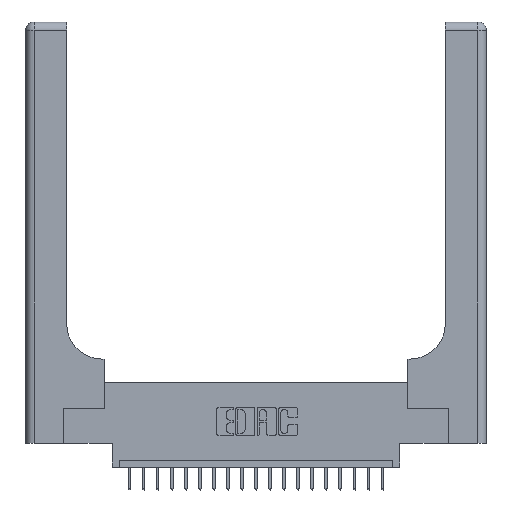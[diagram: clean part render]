
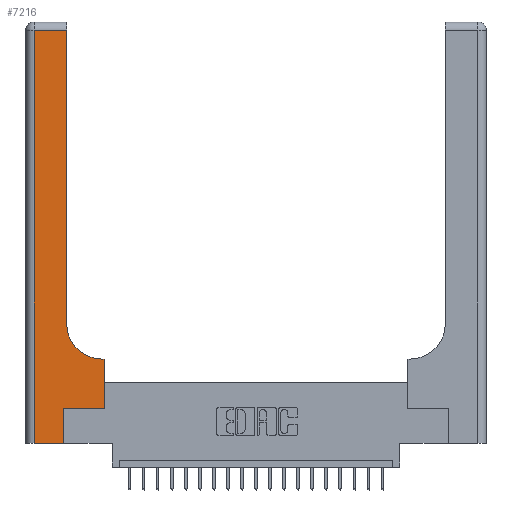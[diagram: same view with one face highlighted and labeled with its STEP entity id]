
A CAD part, top view. The second image highlights one B-rep face of the part: STEP entity #7216.
In plain terms, the highlighted planar face has unit normal (0, 0, 1).
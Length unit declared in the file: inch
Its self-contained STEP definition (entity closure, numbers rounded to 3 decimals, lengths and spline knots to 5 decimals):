
#21 = DIRECTION ( 'NONE',  ( 1., 0., 0. ) ) ;
#581 = CARTESIAN_POINT ( 'NONE',  ( 0.06, 0., 0.37 ) ) ;
#719 = ORIENTED_EDGE ( 'NONE', *, *, #6925, .T. ) ;
#906 = EDGE_CURVE ( 'NONE', #4885, #1287, #16045, .T. ) ;
#971 = DIRECTION ( 'NONE',  ( -1., 0., 0. ) ) ;
#1287 = VERTEX_POINT ( 'NONE', #16649 ) ;
#1726 = DIRECTION ( 'NONE',  ( 1., 0., 0. ) ) ;
#1787 = DIRECTION ( 'NONE',  ( 0., 0., -1. ) ) ;
#2451 = ORIENTED_EDGE ( 'NONE', *, *, #22625, .T. ) ;
#2761 = VECTOR ( 'NONE', #22565, 39.37008 ) ;
#2942 = CARTESIAN_POINT ( 'NONE',  ( 0.2915, 0.6, 0.37 ) ) ;
#3162 = EDGE_CURVE ( 'NONE', #4859, #11652, #18426, .T. ) ;
#3347 = DIRECTION ( 'NONE',  ( 0., 1., 0. ) ) ;
#3668 = VECTOR ( 'NONE', #21945, 39.37008 ) ;
#3741 = CARTESIAN_POINT ( 'NONE',  ( 0.2915, 3., 0.37 ) ) ;
#4030 = ORIENTED_EDGE ( 'NONE', *, *, #906, .T. ) ;
#4605 = VECTOR ( 'NONE', #1726, 39.37008 ) ;
#4859 = VERTEX_POINT ( 'NONE', #581 ) ;
#4885 = VERTEX_POINT ( 'NONE', #20346 ) ;
#5262 = CARTESIAN_POINT ( 'NONE',  ( 0.5585, 0.25, 0.37 ) ) ;
#5513 = DIRECTION ( 'NONE',  ( 0., 1., 0. ) ) ;
#6106 = AXIS2_PLACEMENT_3D ( 'NONE', #15895, #1787, #21 ) ;
#6256 = DIRECTION ( 'NONE',  ( 0., 0., -1. ) ) ;
#6316 = AXIS2_PLACEMENT_3D ( 'NONE', #18442, #6256, #18519 ) ;
#6751 = LINE ( 'NONE', #20317, #16941 ) ;
#6925 = EDGE_CURVE ( 'NONE', #12536, #4859, #7794, .T. ) ;
#7216 = ADVANCED_FACE ( 'NONE', ( #8297 ), #16605, .F. ) ;
#7681 = ORIENTED_EDGE ( 'NONE', *, *, #16705, .T. ) ;
#7794 = LINE ( 'NONE', #8635, #9712 ) ;
#8297 = FACE_OUTER_BOUND ( 'NONE', #13990, .T. ) ;
#8635 = CARTESIAN_POINT ( 'NONE',  ( 0.06, 3., 0.37 ) ) ;
#9516 = VECTOR ( 'NONE', #3347, 39.37008 ) ;
#9712 = VECTOR ( 'NONE', #17436, 39.37008 ) ;
#9859 = LINE ( 'NONE', #19743, #21399 ) ;
#9958 = EDGE_CURVE ( 'NONE', #18834, #12854, #9859, .T. ) ;
#11652 = VERTEX_POINT ( 'NONE', #12809 ) ;
#12324 = CARTESIAN_POINT ( 'NONE',  ( 0.5585, 0.25, 0.37 ) ) ;
#12536 = VERTEX_POINT ( 'NONE', #19107 ) ;
#12741 = ORIENTED_EDGE ( 'NONE', *, *, #22686, .T. ) ;
#12809 = CARTESIAN_POINT ( 'NONE',  ( 0.269, 0., 0.37 ) ) ;
#12854 = VERTEX_POINT ( 'NONE', #5262 ) ;
#12899 = ORIENTED_EDGE ( 'NONE', *, *, #3162, .T. ) ;
#13064 = LINE ( 'NONE', #16672, #3668 ) ;
#13443 = ORIENTED_EDGE ( 'NONE', *, *, #21901, .T. ) ;
#13990 = EDGE_LOOP ( 'NONE', ( #4030, #7681, #719, #12899, #22692, #16936, #13443, #2451, #12741 ) ) ;
#15722 = LINE ( 'NONE', #2942, #2761 ) ;
#15895 = CARTESIAN_POINT ( 'NONE',  ( 0.5415, 0.85, 0.37 ) ) ;
#16045 = LINE ( 'NONE', #3741, #17140 ) ;
#16605 = PLANE ( 'NONE',  #6316 ) ;
#16649 = CARTESIAN_POINT ( 'NONE',  ( 0.2915, 2.94, 0.37 ) ) ;
#16672 = CARTESIAN_POINT ( 'NONE',  ( 0.269, 0., 0.37 ) ) ;
#16705 = EDGE_CURVE ( 'NONE', #1287, #12536, #6751, .T. ) ;
#16936 = ORIENTED_EDGE ( 'NONE', *, *, #9958, .T. ) ;
#16941 = VECTOR ( 'NONE', #971, 39.37008 ) ;
#17140 = VECTOR ( 'NONE', #5513, 39.37008 ) ;
#17436 = DIRECTION ( 'NONE',  ( 0., -1., 0. ) ) ;
#17582 = EDGE_CURVE ( 'NONE', #11652, #18834, #13064, .T. ) ;
#18426 = LINE ( 'NONE', #19493, #4605 ) ;
#18442 = CARTESIAN_POINT ( 'NONE',  ( 0., 3., 0.37 ) ) ;
#18519 = DIRECTION ( 'NONE',  ( -1., 0., 0. ) ) ;
#18661 = CARTESIAN_POINT ( 'NONE',  ( 0.5585, 0.6, 0.37 ) ) ;
#18834 = VERTEX_POINT ( 'NONE', #21458 ) ;
#18895 = CARTESIAN_POINT ( 'NONE',  ( 0.5415, 0.6, 0.37 ) ) ;
#19107 = CARTESIAN_POINT ( 'NONE',  ( 0.06, 2.94, 0.37 ) ) ;
#19493 = CARTESIAN_POINT ( 'NONE',  ( 0., 0., 0.37 ) ) ;
#19545 = VERTEX_POINT ( 'NONE', #18661 ) ;
#19743 = CARTESIAN_POINT ( 'NONE',  ( 0.269, 0.25, 0.37 ) ) ;
#19825 = DIRECTION ( 'NONE',  ( 1., 0., 0. ) ) ;
#19836 = CIRCLE ( 'NONE', #6106, 0.25 ) ;
#20317 = CARTESIAN_POINT ( 'NONE',  ( 0., 2.94, 0.37 ) ) ;
#20346 = CARTESIAN_POINT ( 'NONE',  ( 0.2915, 0.85, 0.37 ) ) ;
#21399 = VECTOR ( 'NONE', #19825, 39.37008 ) ;
#21458 = CARTESIAN_POINT ( 'NONE',  ( 0.269, 0.25, 0.37 ) ) ;
#21608 = LINE ( 'NONE', #12324, #9516 ) ;
#21901 = EDGE_CURVE ( 'NONE', #12854, #19545, #21608, .T. ) ;
#21945 = DIRECTION ( 'NONE',  ( 0., 1., 0. ) ) ;
#22565 = DIRECTION ( 'NONE',  ( -1., 0., 0. ) ) ;
#22625 = EDGE_CURVE ( 'NONE', #19545, #22638, #15722, .T. ) ;
#22638 = VERTEX_POINT ( 'NONE', #18895 ) ;
#22686 = EDGE_CURVE ( 'NONE', #22638, #4885, #19836, .T. ) ;
#22692 = ORIENTED_EDGE ( 'NONE', *, *, #17582, .T. ) ;
